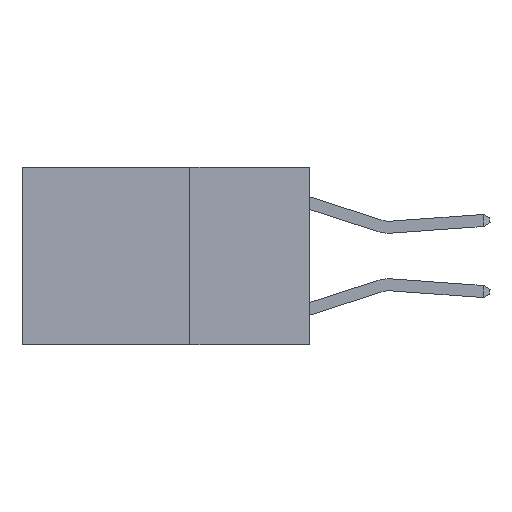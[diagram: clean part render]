
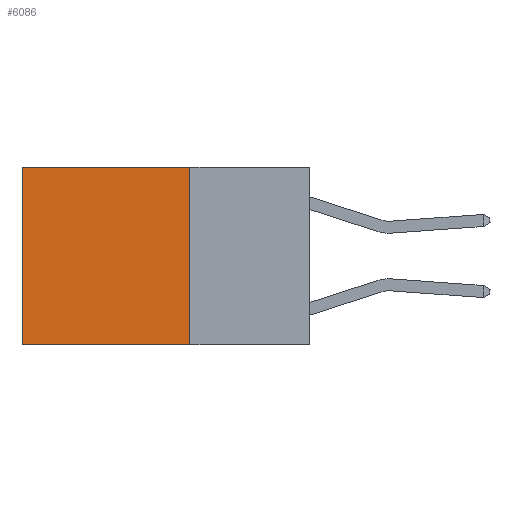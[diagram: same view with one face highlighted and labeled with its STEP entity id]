
A CAD part, left-side view. The second image highlights one B-rep face of the part: STEP entity #6086.
In plain terms, the highlighted planar face has unit normal (-1, 0, 0).
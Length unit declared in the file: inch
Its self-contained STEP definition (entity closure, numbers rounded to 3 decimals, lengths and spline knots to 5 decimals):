
#99 = DIRECTION ( 'NONE',  ( 0., 0., -1. ) ) ;
#154 = EDGE_CURVE ( 'NONE', #11605, #6501, #1130, .T. ) ;
#441 = FACE_OUTER_BOUND ( 'NONE', #873, .T. ) ;
#497 = CARTESIAN_POINT ( 'NONE',  ( 0.2625, 0.6, -0.37 ) ) ;
#647 = AXIS2_PLACEMENT_3D ( 'NONE', #2370, #7157, #1507 ) ;
#873 = EDGE_LOOP ( 'NONE', ( #6758, #3042, #5692, #9805 ) ) ;
#1130 = LINE ( 'NONE', #11375, #4952 ) ;
#1132 = LINE ( 'NONE', #3148, #4179 ) ;
#1507 = DIRECTION ( 'NONE',  ( 0., 0., -1. ) ) ;
#1805 = CARTESIAN_POINT ( 'NONE',  ( 0.2625, 0.25, 0. ) ) ;
#1881 = DIRECTION ( 'NONE',  ( 0., 1., 0. ) ) ;
#1971 = CARTESIAN_POINT ( 'NONE',  ( 0.2625, 0.25, -0.37 ) ) ;
#2370 = CARTESIAN_POINT ( 'NONE',  ( 0.2625, 0.25, 0. ) ) ;
#2436 = PLANE ( 'NONE',  #647 ) ;
#3022 = CARTESIAN_POINT ( 'NONE',  ( 0.2625, 0.25, 0. ) ) ;
#3042 = ORIENTED_EDGE ( 'NONE', *, *, #8456, .F. ) ;
#3148 = CARTESIAN_POINT ( 'NONE',  ( 0.2625, 0.25, 0. ) ) ;
#3629 = EDGE_CURVE ( 'NONE', #5002, #11605, #11133, .T. ) ;
#4111 = VERTEX_POINT ( 'NONE', #1971 ) ;
#4179 = VECTOR ( 'NONE', #4868, 39.37008 ) ;
#4540 = VECTOR ( 'NONE', #1881, 39.37008 ) ;
#4868 = DIRECTION ( 'NONE',  ( 0., 0., -1. ) ) ;
#4952 = VECTOR ( 'NONE', #99, 39.37008 ) ;
#5002 = VERTEX_POINT ( 'NONE', #3022 ) ;
#5531 = CARTESIAN_POINT ( 'NONE',  ( 0.2625, 0.25, -0.37 ) ) ;
#5692 = ORIENTED_EDGE ( 'NONE', *, *, #5908, .F. ) ;
#5908 = EDGE_CURVE ( 'NONE', #5002, #4111, #1132, .T. ) ;
#5948 = CARTESIAN_POINT ( 'NONE',  ( 0.2625, 0.6, 0. ) ) ;
#6086 = ADVANCED_FACE ( 'NONE', ( #441 ), #2436, .F. ) ;
#6501 = VERTEX_POINT ( 'NONE', #497 ) ;
#6758 = ORIENTED_EDGE ( 'NONE', *, *, #154, .T. ) ;
#7157 = DIRECTION ( 'NONE',  ( 1., 0., 0. ) ) ;
#7249 = DIRECTION ( 'NONE',  ( 0., 1., 0. ) ) ;
#8456 = EDGE_CURVE ( 'NONE', #4111, #6501, #9233, .T. ) ;
#9233 = LINE ( 'NONE', #5531, #11839 ) ;
#9805 = ORIENTED_EDGE ( 'NONE', *, *, #3629, .T. ) ;
#11133 = LINE ( 'NONE', #1805, #4540 ) ;
#11375 = CARTESIAN_POINT ( 'NONE',  ( 0.2625, 0.6, 0. ) ) ;
#11605 = VERTEX_POINT ( 'NONE', #5948 ) ;
#11839 = VECTOR ( 'NONE', #7249, 39.37008 ) ;
